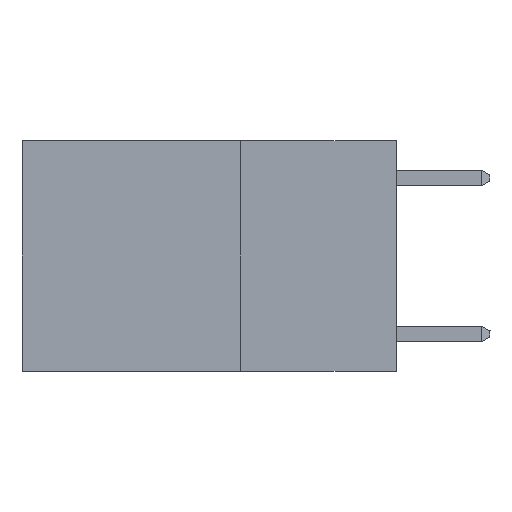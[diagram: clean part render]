
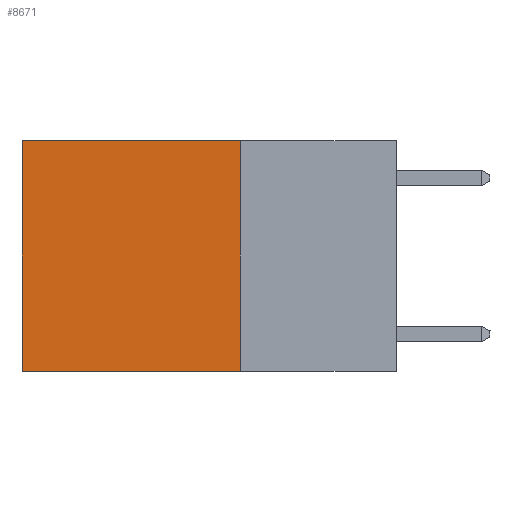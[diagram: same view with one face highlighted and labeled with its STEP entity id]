
A CAD part, left-side view. The second image highlights one B-rep face of the part: STEP entity #8671.
In plain terms, the highlighted planar face has unit normal (-1, 0, 0).
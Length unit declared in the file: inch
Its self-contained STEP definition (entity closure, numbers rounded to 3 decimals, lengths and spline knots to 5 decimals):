
#159 = LINE ( 'NONE', #15209, #13559 ) ;
#221 = EDGE_LOOP ( 'NONE', ( #4497, #10523, #7224, #6351 ) ) ;
#1092 = LINE ( 'NONE', #2487, #11833 ) ;
#1674 = EDGE_CURVE ( 'NONE', #12157, #9125, #10314, .T. ) ;
#2125 = CARTESIAN_POINT ( 'NONE',  ( 0.2625, 0.25, 0. ) ) ;
#2487 = CARTESIAN_POINT ( 'NONE',  ( 0.2625, 0.6, 0. ) ) ;
#2557 = VERTEX_POINT ( 'NONE', #11828 ) ;
#4497 = ORIENTED_EDGE ( 'NONE', *, *, #7007, .T. ) ;
#5548 = CARTESIAN_POINT ( 'NONE',  ( 0.2625, 0.25, 0. ) ) ;
#5745 = DIRECTION ( 'NONE',  ( 0., 1., 0. ) ) ;
#6027 = FACE_OUTER_BOUND ( 'NONE', #221, .T. ) ;
#6351 = ORIENTED_EDGE ( 'NONE', *, *, #1674, .T. ) ;
#6958 = LINE ( 'NONE', #5548, #11742 ) ;
#7007 = EDGE_CURVE ( 'NONE', #9125, #10022, #1092, .T. ) ;
#7224 = ORIENTED_EDGE ( 'NONE', *, *, #9570, .F. ) ;
#7924 = DIRECTION ( 'NONE',  ( 0., 1., 0. ) ) ;
#8376 = CARTESIAN_POINT ( 'NONE',  ( 0.2625, 0.6, 0. ) ) ;
#8671 = ADVANCED_FACE ( 'NONE', ( #6027 ), #11466, .F. ) ;
#9125 = VERTEX_POINT ( 'NONE', #8376 ) ;
#9570 = EDGE_CURVE ( 'NONE', #12157, #2557, #6958, .T. ) ;
#10022 = VERTEX_POINT ( 'NONE', #13572 ) ;
#10314 = LINE ( 'NONE', #14324, #16059 ) ;
#10523 = ORIENTED_EDGE ( 'NONE', *, *, #13763, .F. ) ;
#11466 = PLANE ( 'NONE',  #17347 ) ;
#11742 = VECTOR ( 'NONE', #12418, 39.37008 ) ;
#11828 = CARTESIAN_POINT ( 'NONE',  ( 0.2625, 0.25, -0.37 ) ) ;
#11833 = VECTOR ( 'NONE', #13268, 39.37008 ) ;
#12157 = VERTEX_POINT ( 'NONE', #17272 ) ;
#12418 = DIRECTION ( 'NONE',  ( 0., 0., -1. ) ) ;
#13268 = DIRECTION ( 'NONE',  ( 0., 0., -1. ) ) ;
#13559 = VECTOR ( 'NONE', #5745, 39.37008 ) ;
#13572 = CARTESIAN_POINT ( 'NONE',  ( 0.2625, 0.6, -0.37 ) ) ;
#13763 = EDGE_CURVE ( 'NONE', #2557, #10022, #159, .T. ) ;
#14161 = DIRECTION ( 'NONE',  ( 0., 0., -1. ) ) ;
#14324 = CARTESIAN_POINT ( 'NONE',  ( 0.2625, 0.25, 0. ) ) ;
#15209 = CARTESIAN_POINT ( 'NONE',  ( 0.2625, 0.25, -0.37 ) ) ;
#16059 = VECTOR ( 'NONE', #7924, 39.37008 ) ;
#17084 = DIRECTION ( 'NONE',  ( 1., 0., 0. ) ) ;
#17272 = CARTESIAN_POINT ( 'NONE',  ( 0.2625, 0.25, 0. ) ) ;
#17347 = AXIS2_PLACEMENT_3D ( 'NONE', #2125, #17084, #14161 ) ;
